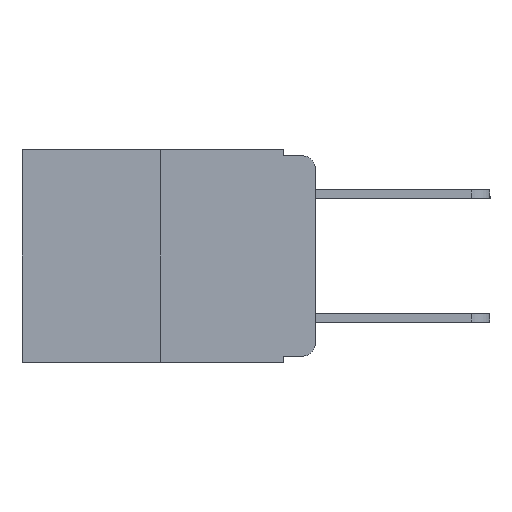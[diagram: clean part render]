
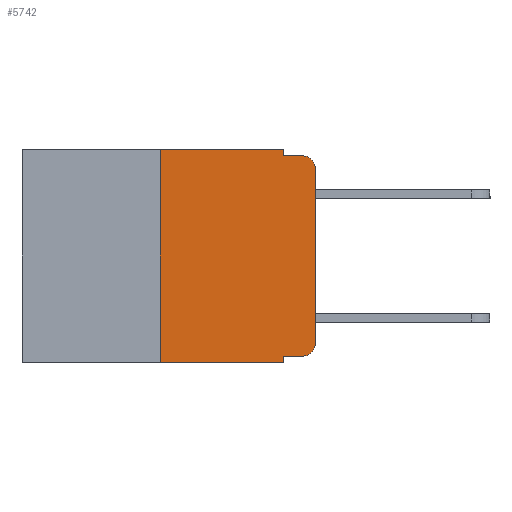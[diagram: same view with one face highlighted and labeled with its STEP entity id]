
A CAD part, left-side view. The second image highlights one B-rep face of the part: STEP entity #5742.
In plain terms, the highlighted planar face has unit normal (-1, 0, 0).
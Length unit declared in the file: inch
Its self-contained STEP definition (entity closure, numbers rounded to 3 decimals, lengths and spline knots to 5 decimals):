
#330 = VERTEX_POINT ( 'NONE', #6582 ) ;
#573 = VECTOR ( 'NONE', #5521, 39.37008 ) ;
#686 = VERTEX_POINT ( 'NONE', #12830 ) ;
#896 = DIRECTION ( 'NONE',  ( 0., -1., 0. ) ) ;
#1187 = VERTEX_POINT ( 'NONE', #8548 ) ;
#1443 = CARTESIAN_POINT ( 'NONE',  ( 0., 0.473, -0.343 ) ) ;
#1828 = CARTESIAN_POINT ( 'NONE',  ( 0., 0.25, 0. ) ) ;
#1841 = CARTESIAN_POINT ( 'NONE',  ( 0., 0.473, 0. ) ) ;
#2352 = LINE ( 'NONE', #4759, #14146 ) ;
#2588 = EDGE_CURVE ( 'NONE', #8102, #13653, #14592, .T. ) ;
#3190 = DIRECTION ( 'NONE',  ( 0., 0., 1. ) ) ;
#3196 = CARTESIAN_POINT ( 'NONE',  ( 0., 0.02, -0.313 ) ) ;
#3556 = EDGE_CURVE ( 'NONE', #686, #14931, #11888, .T. ) ;
#3576 = FACE_OUTER_BOUND ( 'NONE', #11203, .T. ) ;
#3707 = LINE ( 'NONE', #12277, #573 ) ;
#3888 = DIRECTION ( 'NONE',  ( 0., -1., 0. ) ) ;
#4096 = LINE ( 'NONE', #9058, #14897 ) ;
#4474 = DIRECTION ( 'NONE',  ( 0., 0., -1. ) ) ;
#4657 = DIRECTION ( 'NONE',  ( 0., 0., -1. ) ) ;
#4715 = CARTESIAN_POINT ( 'NONE',  ( 0., 0.051, 0. ) ) ;
#4759 = CARTESIAN_POINT ( 'NONE',  ( 0., 0.051, -0.333 ) ) ;
#4785 = CARTESIAN_POINT ( 'NONE',  ( 0., 0.051, 0. ) ) ;
#5521 = DIRECTION ( 'NONE',  ( 0., 0., -1. ) ) ;
#5574 = PLANE ( 'NONE',  #9609 ) ;
#5682 = VECTOR ( 'NONE', #4657, 39.37008 ) ;
#5742 = ADVANCED_FACE ( 'NONE', ( #3576 ), #5574, .F. ) ;
#5750 = EDGE_CURVE ( 'NONE', #1187, #11490, #9753, .T. ) ;
#5884 = VECTOR ( 'NONE', #9806, 39.37008 ) ;
#5905 = CARTESIAN_POINT ( 'NONE',  ( 0., 0.051, -0.343 ) ) ;
#5918 = VECTOR ( 'NONE', #9000, 39.37008 ) ;
#6161 = CARTESIAN_POINT ( 'NONE',  ( 0., 0.02, -0.03 ) ) ;
#6421 = CARTESIAN_POINT ( 'NONE',  ( 0., 0.473, 0. ) ) ;
#6520 = EDGE_CURVE ( 'NONE', #10479, #1187, #2352, .T. ) ;
#6582 = CARTESIAN_POINT ( 'NONE',  ( 0., 0.02, -0.01 ) ) ;
#6753 = DIRECTION ( 'NONE',  ( 1., 0., 0. ) ) ;
#7334 = EDGE_CURVE ( 'NONE', #10479, #14931, #3707, .T. ) ;
#7347 = VERTEX_POINT ( 'NONE', #14420 ) ;
#7375 = DIRECTION ( 'NONE',  ( 0., 0., -1. ) ) ;
#7768 = DIRECTION ( 'NONE',  ( 0., -1., 0. ) ) ;
#7904 = ORIENTED_EDGE ( 'NONE', *, *, #13983, .T. ) ;
#8093 = EDGE_CURVE ( 'NONE', #686, #8102, #14424, .T. ) ;
#8102 = VERTEX_POINT ( 'NONE', #11266 ) ;
#8149 = AXIS2_PLACEMENT_3D ( 'NONE', #6161, #13974, #7375 ) ;
#8162 = CARTESIAN_POINT ( 'NONE',  ( 0., 0.051, -0.01 ) ) ;
#8395 = CARTESIAN_POINT ( 'NONE',  ( 0., 0.051, -0.333 ) ) ;
#8436 = ORIENTED_EDGE ( 'NONE', *, *, #11817, .T. ) ;
#8548 = CARTESIAN_POINT ( 'NONE',  ( 0., 0.02, -0.333 ) ) ;
#8624 = ORIENTED_EDGE ( 'NONE', *, *, #11079, .F. ) ;
#8729 = ORIENTED_EDGE ( 'NONE', *, *, #10336, .F. ) ;
#8790 = ORIENTED_EDGE ( 'NONE', *, *, #2588, .F. ) ;
#8855 = AXIS2_PLACEMENT_3D ( 'NONE', #3196, #11275, #4474 ) ;
#8885 = ORIENTED_EDGE ( 'NONE', *, *, #8093, .F. ) ;
#9000 = DIRECTION ( 'NONE',  ( 0., 0., 1. ) ) ;
#9058 = CARTESIAN_POINT ( 'NONE',  ( 0., 0., 0. ) ) ;
#9090 = ORIENTED_EDGE ( 'NONE', *, *, #3556, .T. ) ;
#9119 = ORIENTED_EDGE ( 'NONE', *, *, #7334, .F. ) ;
#9179 = ORIENTED_EDGE ( 'NONE', *, *, #6520, .T. ) ;
#9307 = ORIENTED_EDGE ( 'NONE', *, *, #5750, .T. ) ;
#9409 = CIRCLE ( 'NONE', #8149, 0.02 ) ;
#9609 = AXIS2_PLACEMENT_3D ( 'NONE', #1841, #6753, #14465 ) ;
#9753 = CIRCLE ( 'NONE', #8855, 0.02 ) ;
#9806 = DIRECTION ( 'NONE',  ( 0., -1., 0. ) ) ;
#10218 = CARTESIAN_POINT ( 'NONE',  ( 0., 0., -0.313 ) ) ;
#10336 = EDGE_CURVE ( 'NONE', #13653, #12343, #14540, .T. ) ;
#10479 = VERTEX_POINT ( 'NONE', #8395 ) ;
#10775 = CARTESIAN_POINT ( 'NONE',  ( 0., 0.051, -0.01 ) ) ;
#11079 = EDGE_CURVE ( 'NONE', #12343, #330, #11140, .T. ) ;
#11140 = LINE ( 'NONE', #10775, #14334 ) ;
#11203 = EDGE_LOOP ( 'NONE', ( #7904, #8436, #8624, #8729, #8790, #8885, #9090, #9119, #9179, #9307 ) ) ;
#11266 = CARTESIAN_POINT ( 'NONE',  ( 0., 0.25, 0. ) ) ;
#11275 = DIRECTION ( 'NONE',  ( -1., 0., 0. ) ) ;
#11409 = VECTOR ( 'NONE', #7768, 39.37008 ) ;
#11490 = VERTEX_POINT ( 'NONE', #10218 ) ;
#11817 = EDGE_CURVE ( 'NONE', #7347, #330, #9409, .T. ) ;
#11888 = LINE ( 'NONE', #1443, #5884 ) ;
#12277 = CARTESIAN_POINT ( 'NONE',  ( 0., 0.051, 0. ) ) ;
#12343 = VERTEX_POINT ( 'NONE', #8162 ) ;
#12830 = CARTESIAN_POINT ( 'NONE',  ( 0., 0.25, -0.343 ) ) ;
#13653 = VERTEX_POINT ( 'NONE', #4785 ) ;
#13974 = DIRECTION ( 'NONE',  ( -1., 0., 0. ) ) ;
#13983 = EDGE_CURVE ( 'NONE', #11490, #7347, #4096, .T. ) ;
#14146 = VECTOR ( 'NONE', #896, 39.37008 ) ;
#14334 = VECTOR ( 'NONE', #3888, 39.37008 ) ;
#14420 = CARTESIAN_POINT ( 'NONE',  ( 0., 0., -0.03 ) ) ;
#14424 = LINE ( 'NONE', #1828, #5918 ) ;
#14465 = DIRECTION ( 'NONE',  ( 0., 0., -1. ) ) ;
#14540 = LINE ( 'NONE', #4715, #5682 ) ;
#14592 = LINE ( 'NONE', #6421, #11409 ) ;
#14897 = VECTOR ( 'NONE', #3190, 39.37008 ) ;
#14931 = VERTEX_POINT ( 'NONE', #5905 ) ;
